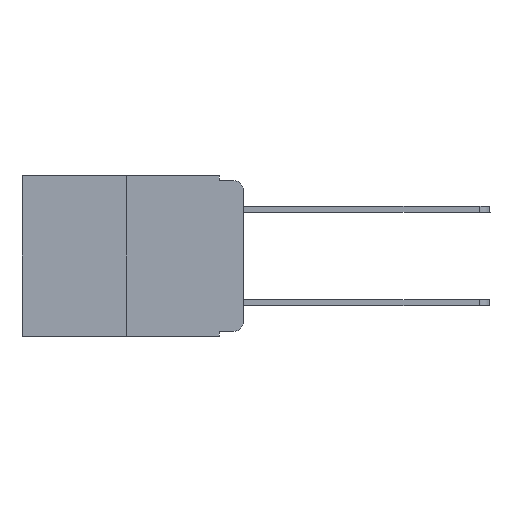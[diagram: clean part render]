
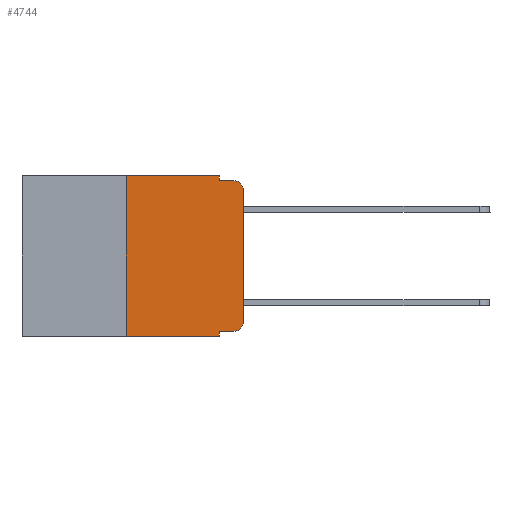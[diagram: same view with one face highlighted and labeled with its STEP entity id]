
A CAD part, left-side view. The second image highlights one B-rep face of the part: STEP entity #4744.
In plain terms, the highlighted planar face has unit normal (-1, 0, 0).
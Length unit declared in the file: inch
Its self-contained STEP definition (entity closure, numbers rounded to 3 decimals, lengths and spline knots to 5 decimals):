
#657 = LINE ( 'NONE', #1556, #6737 ) ;
#745 = CARTESIAN_POINT ( 'NONE',  ( 0., 0.02, -0.333 ) ) ;
#1002 = EDGE_LOOP ( 'NONE', ( #8070, #13227, #10515, #2978, #9175, #14158, #16558, #20666, #20087, #13820 ) ) ;
#1037 = CARTESIAN_POINT ( 'NONE',  ( 0., 0.051, -0.01 ) ) ;
#1304 = CARTESIAN_POINT ( 'NONE',  ( 0., 0.02, -0.313 ) ) ;
#1556 = CARTESIAN_POINT ( 'NONE',  ( 0., 0.473, 0. ) ) ;
#1585 = DIRECTION ( 'NONE',  ( 0., 0., -1. ) ) ;
#2069 = CARTESIAN_POINT ( 'NONE',  ( 0., 0.02, -0.03 ) ) ;
#2325 = AXIS2_PLACEMENT_3D ( 'NONE', #7700, #15974, #9451 ) ;
#2347 = VERTEX_POINT ( 'NONE', #5387 ) ;
#2410 = CIRCLE ( 'NONE', #16450, 0.02 ) ;
#2579 = VERTEX_POINT ( 'NONE', #7625 ) ;
#2592 = DIRECTION ( 'NONE',  ( 0., -1., 0. ) ) ;
#2978 = ORIENTED_EDGE ( 'NONE', *, *, #14790, .F. ) ;
#4307 = LINE ( 'NONE', #5687, #18457 ) ;
#4744 = ADVANCED_FACE ( 'NONE', ( #11315 ), #20667, .F. ) ;
#4758 = DIRECTION ( 'NONE',  ( -1., 0., 0. ) ) ;
#4836 = CARTESIAN_POINT ( 'NONE',  ( 0., 0.051, 0. ) ) ;
#5168 = VERTEX_POINT ( 'NONE', #10066 ) ;
#5387 = CARTESIAN_POINT ( 'NONE',  ( 0., 0.02, -0.01 ) ) ;
#5687 = CARTESIAN_POINT ( 'NONE',  ( 0., 0., 0. ) ) ;
#6730 = VERTEX_POINT ( 'NONE', #19315 ) ;
#6737 = VECTOR ( 'NONE', #15891, 39.37008 ) ;
#7201 = VERTEX_POINT ( 'NONE', #19062 ) ;
#7596 = LINE ( 'NONE', #12645, #8843 ) ;
#7625 = CARTESIAN_POINT ( 'NONE',  ( 0., 0.051, -0.333 ) ) ;
#7639 = DIRECTION ( 'NONE',  ( 0., -1., 0. ) ) ;
#7700 = CARTESIAN_POINT ( 'NONE',  ( 0., 0.473, 0. ) ) ;
#7815 = LINE ( 'NONE', #10616, #9832 ) ;
#8070 = ORIENTED_EDGE ( 'NONE', *, *, #8831, .T. ) ;
#8412 = DIRECTION ( 'NONE',  ( 0., 0., 1. ) ) ;
#8495 = VECTOR ( 'NONE', #17512, 39.37008 ) ;
#8831 = EDGE_CURVE ( 'NONE', #15090, #5168, #4307, .T. ) ;
#8843 = VECTOR ( 'NONE', #7639, 39.37008 ) ;
#8932 = DIRECTION ( 'NONE',  ( 0., 0., -1. ) ) ;
#8974 = DIRECTION ( 'NONE',  ( 0., 0., 1. ) ) ;
#8978 = EDGE_CURVE ( 'NONE', #19022, #14374, #7596, .T. ) ;
#9175 = ORIENTED_EDGE ( 'NONE', *, *, #17276, .F. ) ;
#9451 = DIRECTION ( 'NONE',  ( 0., 0., -1. ) ) ;
#9757 = LINE ( 'NONE', #4836, #8495 ) ;
#9832 = VECTOR ( 'NONE', #8932, 39.37008 ) ;
#10066 = CARTESIAN_POINT ( 'NONE',  ( 0., 0., -0.03 ) ) ;
#10381 = VERTEX_POINT ( 'NONE', #18992 ) ;
#10481 = LINE ( 'NONE', #1037, #12507 ) ;
#10515 = ORIENTED_EDGE ( 'NONE', *, *, #17845, .F. ) ;
#10578 = CARTESIAN_POINT ( 'NONE',  ( 0., 0.25, -0.343 ) ) ;
#10616 = CARTESIAN_POINT ( 'NONE',  ( 0., 0.051, 0. ) ) ;
#11309 = CARTESIAN_POINT ( 'NONE',  ( 0., 0.25, 0. ) ) ;
#11315 = FACE_OUTER_BOUND ( 'NONE', #1002, .T. ) ;
#11862 = EDGE_CURVE ( 'NONE', #19656, #15090, #2410, .T. ) ;
#12003 = VECTOR ( 'NONE', #8412, 39.37008 ) ;
#12053 = EDGE_CURVE ( 'NONE', #19022, #7201, #13987, .T. ) ;
#12507 = VECTOR ( 'NONE', #2592, 39.37008 ) ;
#12645 = CARTESIAN_POINT ( 'NONE',  ( 0., 0.473, -0.343 ) ) ;
#13170 = AXIS2_PLACEMENT_3D ( 'NONE', #2069, #16228, #19583 ) ;
#13227 = ORIENTED_EDGE ( 'NONE', *, *, #18202, .T. ) ;
#13738 = EDGE_CURVE ( 'NONE', #2579, #19656, #14398, .T. ) ;
#13820 = ORIENTED_EDGE ( 'NONE', *, *, #11862, .T. ) ;
#13987 = LINE ( 'NONE', #11309, #12003 ) ;
#14158 = ORIENTED_EDGE ( 'NONE', *, *, #12053, .F. ) ;
#14374 = VERTEX_POINT ( 'NONE', #15884 ) ;
#14398 = LINE ( 'NONE', #16128, #16150 ) ;
#14790 = EDGE_CURVE ( 'NONE', #10381, #6730, #7815, .T. ) ;
#15090 = VERTEX_POINT ( 'NONE', #19855 ) ;
#15884 = CARTESIAN_POINT ( 'NONE',  ( 0., 0.051, -0.343 ) ) ;
#15891 = DIRECTION ( 'NONE',  ( 0., -1., 0. ) ) ;
#15974 = DIRECTION ( 'NONE',  ( 1., 0., 0. ) ) ;
#16128 = CARTESIAN_POINT ( 'NONE',  ( 0., 0.051, -0.333 ) ) ;
#16150 = VECTOR ( 'NONE', #16206, 39.37008 ) ;
#16206 = DIRECTION ( 'NONE',  ( 0., -1., 0. ) ) ;
#16228 = DIRECTION ( 'NONE',  ( -1., 0., 0. ) ) ;
#16420 = EDGE_CURVE ( 'NONE', #2579, #14374, #9757, .T. ) ;
#16450 = AXIS2_PLACEMENT_3D ( 'NONE', #1304, #4758, #1585 ) ;
#16558 = ORIENTED_EDGE ( 'NONE', *, *, #8978, .T. ) ;
#17276 = EDGE_CURVE ( 'NONE', #7201, #10381, #657, .T. ) ;
#17512 = DIRECTION ( 'NONE',  ( 0., 0., -1. ) ) ;
#17845 = EDGE_CURVE ( 'NONE', #6730, #2347, #10481, .T. ) ;
#18202 = EDGE_CURVE ( 'NONE', #5168, #2347, #18801, .T. ) ;
#18457 = VECTOR ( 'NONE', #8974, 39.37008 ) ;
#18801 = CIRCLE ( 'NONE', #13170, 0.02 ) ;
#18992 = CARTESIAN_POINT ( 'NONE',  ( 0., 0.051, 0. ) ) ;
#19022 = VERTEX_POINT ( 'NONE', #10578 ) ;
#19062 = CARTESIAN_POINT ( 'NONE',  ( 0., 0.25, 0. ) ) ;
#19315 = CARTESIAN_POINT ( 'NONE',  ( 0., 0.051, -0.01 ) ) ;
#19583 = DIRECTION ( 'NONE',  ( 0., 0., -1. ) ) ;
#19656 = VERTEX_POINT ( 'NONE', #745 ) ;
#19855 = CARTESIAN_POINT ( 'NONE',  ( 0., 0., -0.313 ) ) ;
#20087 = ORIENTED_EDGE ( 'NONE', *, *, #13738, .T. ) ;
#20666 = ORIENTED_EDGE ( 'NONE', *, *, #16420, .F. ) ;
#20667 = PLANE ( 'NONE',  #2325 ) ;
